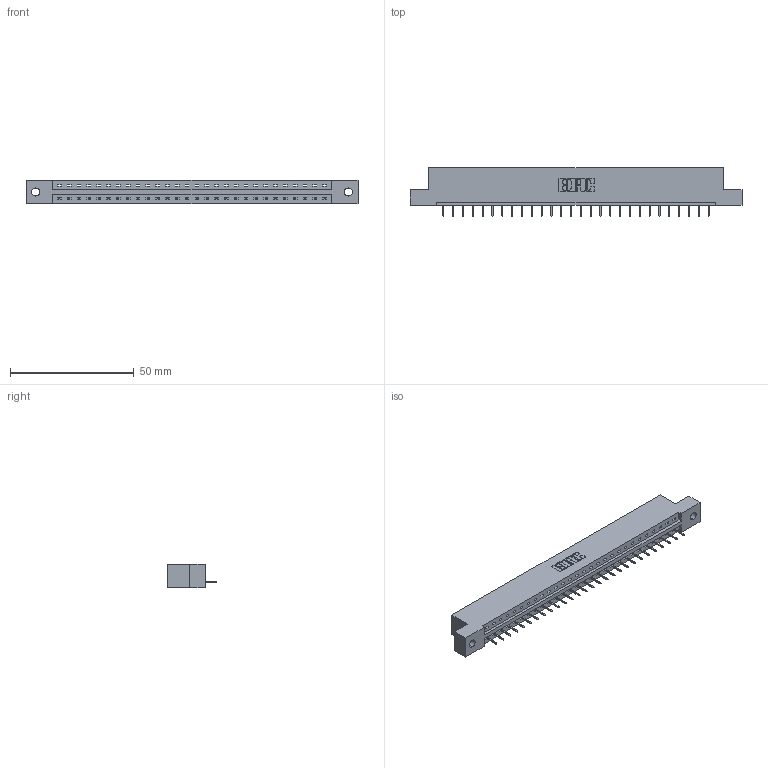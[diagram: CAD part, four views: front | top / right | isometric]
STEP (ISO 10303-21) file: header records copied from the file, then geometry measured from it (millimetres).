
FILE_DESCRIPTION (( 'STEP AP203' ), '1' );
FILE_NAME ('337-028-524-102.STEP', '2018-08-06T09:59:27', ( '' ), ( '' ), 'SwSTEP 2.0', 'SolidWorks 2016', '' );
FILE_SCHEMA (( 'CONFIG_CONTROL_DESIGN' ));
Length unit declared in the file: inch
Products named in the file (3): 337-028-524-102; 337 Part_Flush Mounting Lugs - 0.128 Dia; 345-292-001_345-293-124
Assembly tree (29 placements, depth 2):
  337-028-524-102
    337 Part_Flush Mounting Lugs - 0.128 Dia
    345-292-001_345-293-124  x28
Bounding box: 133.96 x 19.69 x 9.4 mm (x, y, z)
Volume: 13600.4 mm3; surface area: 13317.4 mm2
Topology: 29 solids, 29 shells, 1962 faces, 5687 edges, 3678 vertices
Faces by surface type: plane 1526, cylinder 436
Entity records: 22701 total; most frequent: CARTESIAN_POINT 3958, ORIENTED_EDGE 3922, DIRECTION 3361, EDGE_CURVE 1961, VECTOR 1837, LINE 1837, VERTEX_POINT 1302, AXIS2_PLACEMENT_3D 762
